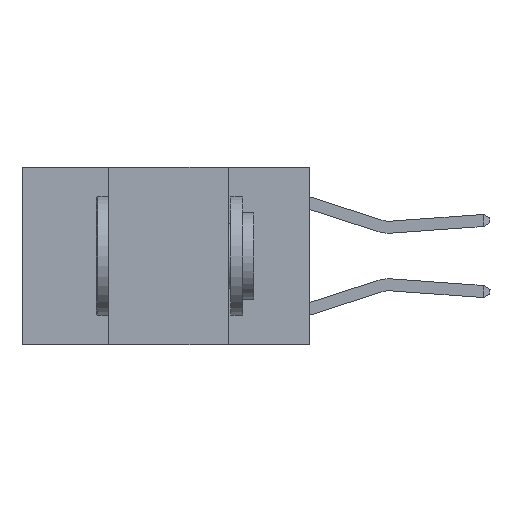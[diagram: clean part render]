
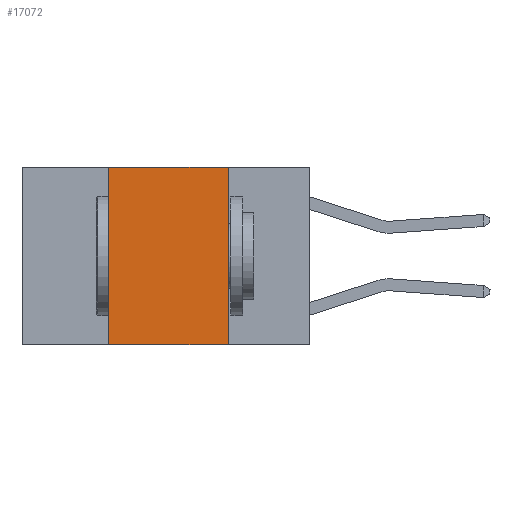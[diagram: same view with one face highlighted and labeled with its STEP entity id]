
A CAD part, left-side view. The second image highlights one B-rep face of the part: STEP entity #17072.
In plain terms, the highlighted planar face has unit normal (-1, 0, 0).
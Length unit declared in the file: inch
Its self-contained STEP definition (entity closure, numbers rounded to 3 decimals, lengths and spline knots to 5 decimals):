
#66 = VERTEX_POINT ( 'NONE', #13938 ) ;
#994 = VERTEX_POINT ( 'NONE', #16396 ) ;
#1572 = LINE ( 'NONE', #19623, #10440 ) ;
#3129 = EDGE_CURVE ( 'NONE', #21535, #19224, #1572, .T. ) ;
#3737 = VECTOR ( 'NONE', #15976, 39.37008 ) ;
#7988 = DIRECTION ( 'NONE',  ( 0., -1., 0. ) ) ;
#9114 = DIRECTION ( 'NONE',  ( 0., -1., 0. ) ) ;
#10216 = DIRECTION ( 'NONE',  ( 0., 0., -1. ) ) ;
#10440 = VECTOR ( 'NONE', #7988, 39.37008 ) ;
#10835 = FACE_OUTER_BOUND ( 'NONE', #18936, .T. ) ;
#11470 = VECTOR ( 'NONE', #9114, 39.37008 ) ;
#12104 = AXIS2_PLACEMENT_3D ( 'NONE', #16844, #20167, #10216 ) ;
#12210 = ORIENTED_EDGE ( 'NONE', *, *, #16708, .F. ) ;
#12737 = ORIENTED_EDGE ( 'NONE', *, *, #20030, .F. ) ;
#13236 = CARTESIAN_POINT ( 'NONE',  ( 0., 0.42, 0. ) ) ;
#13938 = CARTESIAN_POINT ( 'NONE',  ( 0., 0.17, -0.37 ) ) ;
#14091 = CARTESIAN_POINT ( 'NONE',  ( 0., 0.6, -0.37 ) ) ;
#14152 = VECTOR ( 'NONE', #14966, 39.37008 ) ;
#14333 = CARTESIAN_POINT ( 'NONE',  ( 0., 0.17, 0. ) ) ;
#14966 = DIRECTION ( 'NONE',  ( 0., 0., 1. ) ) ;
#15178 = PLANE ( 'NONE',  #12104 ) ;
#15399 = LINE ( 'NONE', #14091, #11470 ) ;
#15833 = ORIENTED_EDGE ( 'NONE', *, *, #21166, .T. ) ;
#15976 = DIRECTION ( 'NONE',  ( 0., 0., -1. ) ) ;
#16396 = CARTESIAN_POINT ( 'NONE',  ( 0., 0.42, -0.37 ) ) ;
#16626 = ORIENTED_EDGE ( 'NONE', *, *, #3129, .F. ) ;
#16673 = CARTESIAN_POINT ( 'NONE',  ( 0., 0.42, 0. ) ) ;
#16708 = EDGE_CURVE ( 'NONE', #19224, #66, #20926, .T. ) ;
#16844 = CARTESIAN_POINT ( 'NONE',  ( 0., 0.6, 0. ) ) ;
#17072 = ADVANCED_FACE ( 'NONE', ( #10835 ), #15178, .F. ) ;
#18936 = EDGE_LOOP ( 'NONE', ( #12210, #16626, #12737, #15833 ) ) ;
#19087 = LINE ( 'NONE', #13236, #14152 ) ;
#19224 = VERTEX_POINT ( 'NONE', #21172 ) ;
#19623 = CARTESIAN_POINT ( 'NONE',  ( 0., 0.6, 0. ) ) ;
#20030 = EDGE_CURVE ( 'NONE', #994, #21535, #19087, .T. ) ;
#20167 = DIRECTION ( 'NONE',  ( 1., 0., 0. ) ) ;
#20926 = LINE ( 'NONE', #14333, #3737 ) ;
#21166 = EDGE_CURVE ( 'NONE', #994, #66, #15399, .T. ) ;
#21172 = CARTESIAN_POINT ( 'NONE',  ( 0., 0.17, 0. ) ) ;
#21535 = VERTEX_POINT ( 'NONE', #16673 ) ;
